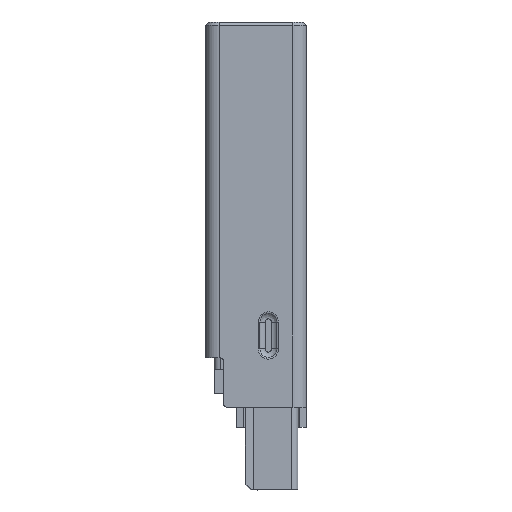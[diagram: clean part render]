
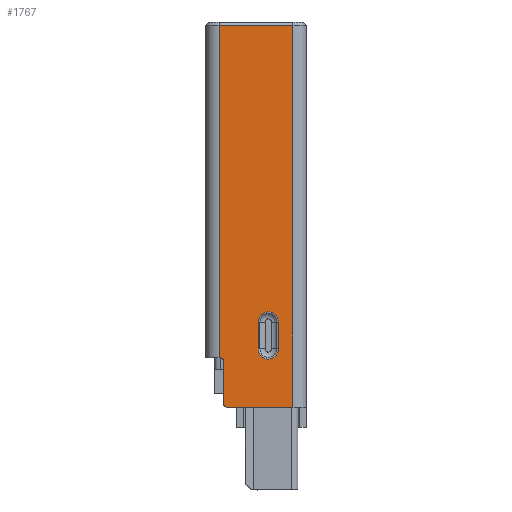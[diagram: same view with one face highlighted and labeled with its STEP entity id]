
A CAD part, left-side view. The second image highlights one B-rep face of the part: STEP entity #1767.
In plain terms, the highlighted planar face has unit normal (-1, 0, 0).
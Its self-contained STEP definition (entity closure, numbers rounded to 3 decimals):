
#550 = CARTESIAN_POINT ( 'NONE',  ( -6., -1.002, -14.6 ) ) ;
#737 = DIRECTION ( 'NONE',  ( 0., 0., -1. ) ) ;
#861 = VERTEX_POINT ( 'NONE', #21476 ) ;
#949 = VERTEX_POINT ( 'NONE', #6446 ) ;
#1044 = DIRECTION ( 'NONE',  ( 0., 1., 0. ) ) ;
#1046 = EDGE_CURVE ( 'NONE', #7832, #2013, #8327, .T. ) ;
#1297 = CARTESIAN_POINT ( 'NONE',  ( -6., -1.002, -14.6 ) ) ;
#1456 = EDGE_CURVE ( 'NONE', #14625, #26402, #27710, .T. ) ;
#1553 = EDGE_CURVE ( 'NONE', #2013, #20218, #7521, .T. ) ;
#1710 = LINE ( 'NONE', #10016, #3086 ) ;
#1767 = ADVANCED_FACE ( 'NONE', ( #3944, #3661 ), #16811, .F. ) ;
#1802 = CARTESIAN_POINT ( 'NONE',  ( -6., -1.716, 0.191 ) ) ;
#2013 = VERTEX_POINT ( 'NONE', #1297 ) ;
#3086 = VECTOR ( 'NONE', #14578, 1000. ) ;
#3133 = VERTEX_POINT ( 'NONE', #12051 ) ;
#3541 = CARTESIAN_POINT ( 'NONE',  ( -6., 1.45, -8.675 ) ) ;
#3549 = VERTEX_POINT ( 'NONE', #16315 ) ;
#3661 = FACE_OUTER_BOUND ( 'NONE', #28142, .T. ) ;
#3683 = CIRCLE ( 'NONE', #19690, 0.15 ) ;
#3944 = FACE_BOUND ( 'NONE', #15592, .T. ) ;
#3975 = DIRECTION ( 'NONE',  ( 0., 0., -1. ) ) ;
#4487 = CARTESIAN_POINT ( 'NONE',  ( -6., -0.098, -14.6 ) ) ;
#4539 = VECTOR ( 'NONE', #737, 1000. ) ;
#5254 = CARTESIAN_POINT ( 'NONE',  ( -6., -0.098, -14.6 ) ) ;
#5365 = CARTESIAN_POINT ( 'NONE',  ( -6., -1.002, -13.4 ) ) ;
#5628 = CARTESIAN_POINT ( 'NONE',  ( -6., -1.002, -13.4 ) ) ;
#6119 = LINE ( 'NONE', #23576, #13632 ) ;
#6196 = EDGE_CURVE ( 'NONE', #12183, #14426, #18241, .T. ) ;
#6211 = EDGE_CURVE ( 'NONE', #20218, #949, #18755, .T. ) ;
#6446 = CARTESIAN_POINT ( 'NONE',  ( -6., -0.098, -13.4 ) ) ;
#6827 = ORIENTED_EDGE ( 'NONE', *, *, #21233, .T. ) ;
#6925 = CARTESIAN_POINT ( 'NONE',  ( -6., -1.65, -17.2 ) ) ;
#6971 = CARTESIAN_POINT ( 'NONE',  ( -6., 1.45, -17.05 ) ) ;
#6999 = CARTESIAN_POINT ( 'NONE',  ( -6., -0.098, -14.6 ) ) ;
#7404 = ORIENTED_EDGE ( 'NONE', *, *, #20633, .F. ) ;
#7521 = LINE ( 'NONE', #24705, #19243 ) ;
#7719 = ORIENTED_EDGE ( 'NONE', *, *, #12503, .F. ) ;
#7832 = VERTEX_POINT ( 'NONE', #5254 ) ;
#8294 = DIRECTION ( 'NONE',  ( 0., 1., 0. ) ) ;
#8327 =( BOUNDED_CURVE ( )  B_SPLINE_CURVE ( 3, ( #6999, #11424, #13288, #22050, #13559, #26327, #550 ),
 .UNSPECIFIED., .F., .F. ) 
 B_SPLINE_CURVE_WITH_KNOTS ( ( 4, 3, 4 ),
 ( 0., 0.5, 1. ),
 .UNSPECIFIED. ) 
 CURVE ( )  GEOMETRIC_REPRESENTATION_ITEM ( )  RATIONAL_B_SPLINE_CURVE ( ( 1., 0.805, 0.805, 1., 0.805, 0.805, 1. ) ) 
 REPRESENTATION_ITEM ( '' )  );
#8537 = ORIENTED_EDGE ( 'NONE', *, *, #6196, .F. ) ;
#9518 = CARTESIAN_POINT ( 'NONE',  ( -6., -0.098, -12.495 ) ) ;
#10016 = CARTESIAN_POINT ( 'NONE',  ( -6., 0., -0.15 ) ) ;
#10558 = EDGE_CURVE ( 'NONE', #10700, #3133, #12991, .T. ) ;
#10700 = VERTEX_POINT ( 'NONE', #6925 ) ;
#11424 = CARTESIAN_POINT ( 'NONE',  ( -6., -0.098, -14.865 ) ) ;
#11527 = DIRECTION ( 'NONE',  ( 0., 0., 1. ) ) ;
#12050 = CARTESIAN_POINT ( 'NONE',  ( -6., 1.3, -17.05 ) ) ;
#12051 = CARTESIAN_POINT ( 'NONE',  ( -6., 1.3, -17.2 ) ) ;
#12183 = VERTEX_POINT ( 'NONE', #24369 ) ;
#12503 = EDGE_CURVE ( 'NONE', #26402, #12183, #3683, .T. ) ;
#12617 = LINE ( 'NONE', #4487, #22308 ) ;
#12991 = LINE ( 'NONE', #14860, #16829 ) ;
#13277 = ORIENTED_EDGE ( 'NONE', *, *, #1553, .F. ) ;
#13288 = CARTESIAN_POINT ( 'NONE',  ( -6., -0.285, -15.052 ) ) ;
#13559 = CARTESIAN_POINT ( 'NONE',  ( -6., -0.815, -15.052 ) ) ;
#13632 = VECTOR ( 'NONE', #3975, 1000. ) ;
#14162 = CARTESIAN_POINT ( 'NONE',  ( -6., 1.6, -15.15 ) ) ;
#14363 = CARTESIAN_POINT ( 'NONE',  ( -6., 0., -15. ) ) ;
#14426 = VERTEX_POINT ( 'NONE', #18611 ) ;
#14503 = AXIS2_PLACEMENT_3D ( 'NONE', #12050, #20661, #1044 ) ;
#14578 = DIRECTION ( 'NONE',  ( 0., -1., 0. ) ) ;
#14625 = VERTEX_POINT ( 'NONE', #6971 ) ;
#14860 = CARTESIAN_POINT ( 'NONE',  ( -6., 0., -17.2 ) ) ;
#14955 = DIRECTION ( 'NONE',  ( 1., 0., 0. ) ) ;
#15132 = EDGE_CURVE ( 'NONE', #3133, #14625, #26853, .T. ) ;
#15216 = DIRECTION ( 'NONE',  ( 0., 0., -1. ) ) ;
#15348 = EDGE_CURVE ( 'NONE', #949, #7832, #12617, .T. ) ;
#15592 = EDGE_LOOP ( 'NONE', ( #13277, #22142, #16464, #16115 ) ) ;
#16115 = ORIENTED_EDGE ( 'NONE', *, *, #6211, .F. ) ;
#16315 = CARTESIAN_POINT ( 'NONE',  ( -6., 1.65, -0.15 ) ) ;
#16464 = ORIENTED_EDGE ( 'NONE', *, *, #15348, .F. ) ;
#16529 = DIRECTION ( 'NONE',  ( 0., 0., -1. ) ) ;
#16811 = PLANE ( 'NONE',  #20650 ) ;
#16829 = VECTOR ( 'NONE', #8294, 1000. ) ;
#17812 = ORIENTED_EDGE ( 'NONE', *, *, #1456, .F. ) ;
#18041 = CARTESIAN_POINT ( 'NONE',  ( -6., 1.45, -15.15 ) ) ;
#18241 = LINE ( 'NONE', #14363, #20748 ) ;
#18283 = EDGE_CURVE ( 'NONE', #3549, #861, #1710, .T. ) ;
#18611 = CARTESIAN_POINT ( 'NONE',  ( -6., 1.65, -15. ) ) ;
#18755 =( BOUNDED_CURVE ( )  B_SPLINE_CURVE ( 3, ( #5365, #24832, #9518, #20679 ),
 .UNSPECIFIED., .F., .F. ) 
 B_SPLINE_CURVE_WITH_KNOTS ( ( 4, 4 ),
 ( 0., 1. ),
 .UNSPECIFIED. ) 
 CURVE ( )  GEOMETRIC_REPRESENTATION_ITEM ( )  RATIONAL_B_SPLINE_CURVE ( ( 1., 0.333, 0.333, 1. ) ) 
 REPRESENTATION_ITEM ( '' )  );
#19135 = DIRECTION ( 'NONE',  ( 0., 0., 1. ) ) ;
#19243 = VECTOR ( 'NONE', #11527, 1000. ) ;
#19287 = ORIENTED_EDGE ( 'NONE', *, *, #10558, .F. ) ;
#19690 = AXIS2_PLACEMENT_3D ( 'NONE', #14162, #23190, #27479 ) ;
#20067 = ORIENTED_EDGE ( 'NONE', *, *, #18283, .F. ) ;
#20218 = VERTEX_POINT ( 'NONE', #5628 ) ;
#20633 = EDGE_CURVE ( 'NONE', #861, #10700, #6119, .T. ) ;
#20650 = AXIS2_PLACEMENT_3D ( 'NONE', #1802, #14955, #16529 ) ;
#20661 = DIRECTION ( 'NONE',  ( 1., 0., 0. ) ) ;
#20679 = CARTESIAN_POINT ( 'NONE',  ( -6., -0.098, -13.4 ) ) ;
#20748 = VECTOR ( 'NONE', #25252, 1000. ) ;
#21233 = EDGE_CURVE ( 'NONE', #3549, #14426, #26935, .T. ) ;
#21476 = CARTESIAN_POINT ( 'NONE',  ( -6., -1.65, -0.15 ) ) ;
#22050 = CARTESIAN_POINT ( 'NONE',  ( -6., -0.55, -15.052 ) ) ;
#22142 = ORIENTED_EDGE ( 'NONE', *, *, #1046, .F. ) ;
#22308 = VECTOR ( 'NONE', #15216, 1000. ) ;
#22517 = CARTESIAN_POINT ( 'NONE',  ( -6., 1.65, 0.191 ) ) ;
#23190 = DIRECTION ( 'NONE',  ( -1., 0., 0. ) ) ;
#23576 = CARTESIAN_POINT ( 'NONE',  ( -6., -1.65, -8.675 ) ) ;
#24369 = CARTESIAN_POINT ( 'NONE',  ( -6., 1.6, -15. ) ) ;
#24705 = CARTESIAN_POINT ( 'NONE',  ( -6., -1.002, -8.675 ) ) ;
#24832 = CARTESIAN_POINT ( 'NONE',  ( -6., -1.002, -12.495 ) ) ;
#25252 = DIRECTION ( 'NONE',  ( 0., 1., 0. ) ) ;
#26327 = CARTESIAN_POINT ( 'NONE',  ( -6., -1.002, -14.865 ) ) ;
#26402 = VERTEX_POINT ( 'NONE', #18041 ) ;
#26776 = ORIENTED_EDGE ( 'NONE', *, *, #15132, .F. ) ;
#26853 = CIRCLE ( 'NONE', #14503, 0.15 ) ;
#26935 = LINE ( 'NONE', #22517, #4539 ) ;
#27479 = DIRECTION ( 'NONE',  ( 0., 1., 0. ) ) ;
#27710 = LINE ( 'NONE', #3541, #27819 ) ;
#27819 = VECTOR ( 'NONE', #19135, 1000. ) ;
#28142 = EDGE_LOOP ( 'NONE', ( #19287, #7404, #20067, #6827, #8537, #7719, #17812, #26776 ) ) ;
